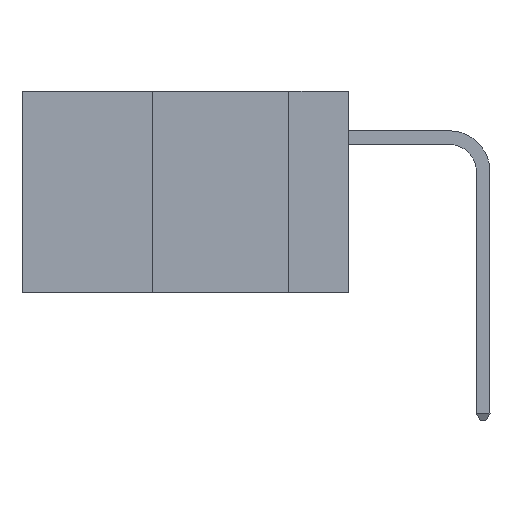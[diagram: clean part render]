
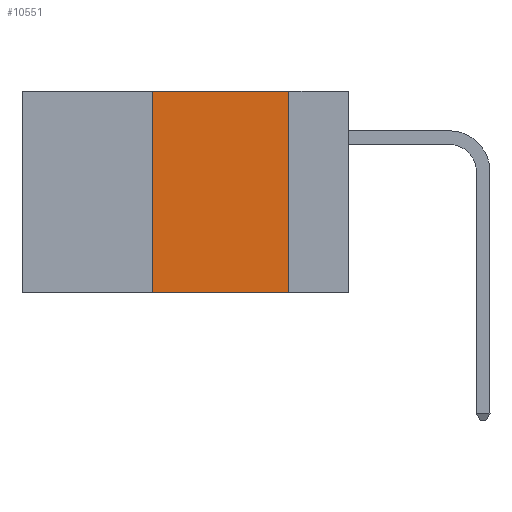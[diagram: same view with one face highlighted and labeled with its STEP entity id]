
A CAD part, left-side view. The second image highlights one B-rep face of the part: STEP entity #10551.
In plain terms, the highlighted planar face has unit normal (-1, 0, 0).
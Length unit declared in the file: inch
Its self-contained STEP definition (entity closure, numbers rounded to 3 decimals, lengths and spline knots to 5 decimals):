
#2004 = VERTEX_POINT ( 'NONE', #26860 ) ;
#2212 = EDGE_CURVE ( 'NONE', #38473, #3203, #31771, .T. ) ;
#3203 = VERTEX_POINT ( 'NONE', #31672 ) ;
#3282 = EDGE_CURVE ( 'NONE', #30031, #2004, #11717, .T. ) ;
#3926 = EDGE_CURVE ( 'NONE', #38473, #30031, #19703, .T. ) ;
#5489 = CARTESIAN_POINT ( 'NONE',  ( 0., 0.11, 0. ) ) ;
#5500 = DIRECTION ( 'NONE',  ( 0., -1., 0. ) ) ;
#5546 = CARTESIAN_POINT ( 'NONE',  ( 0., 0.36, -0.37 ) ) ;
#6443 = PLANE ( 'NONE',  #30149 ) ;
#7255 = ORIENTED_EDGE ( 'NONE', *, *, #3282, .F. ) ;
#7257 = CARTESIAN_POINT ( 'NONE',  ( 0., 0.36, 0. ) ) ;
#8754 = VECTOR ( 'NONE', #25417, 39.37008 ) ;
#10551 = ADVANCED_FACE ( 'NONE', ( #21468 ), #6443, .F. ) ;
#11430 = CARTESIAN_POINT ( 'NONE',  ( 0., 0.6, -0.37 ) ) ;
#11717 = LINE ( 'NONE', #24358, #22481 ) ;
#12381 = CARTESIAN_POINT ( 'NONE',  ( 0., 0.6, 0. ) ) ;
#15226 = ORIENTED_EDGE ( 'NONE', *, *, #2212, .T. ) ;
#18297 = EDGE_LOOP ( 'NONE', ( #26892, #7255, #31265, #15226 ) ) ;
#19703 = LINE ( 'NONE', #7257, #8754 ) ;
#21468 = FACE_OUTER_BOUND ( 'NONE', #18297, .T. ) ;
#21863 = DIRECTION ( 'NONE',  ( 0., 0., -1. ) ) ;
#22481 = VECTOR ( 'NONE', #38576, 39.37008 ) ;
#22729 = CARTESIAN_POINT ( 'NONE',  ( 0., 0.36, 0. ) ) ;
#24358 = CARTESIAN_POINT ( 'NONE',  ( 0., 0.6, 0. ) ) ;
#25417 = DIRECTION ( 'NONE',  ( 0., 0., 1. ) ) ;
#26860 = CARTESIAN_POINT ( 'NONE',  ( 0., 0.11, 0. ) ) ;
#26892 = ORIENTED_EDGE ( 'NONE', *, *, #28267, .F. ) ;
#28267 = EDGE_CURVE ( 'NONE', #2004, #3203, #35875, .T. ) ;
#30031 = VERTEX_POINT ( 'NONE', #22729 ) ;
#30147 = DIRECTION ( 'NONE',  ( 1., 0., 0. ) ) ;
#30149 = AXIS2_PLACEMENT_3D ( 'NONE', #12381, #30147, #21863 ) ;
#31265 = ORIENTED_EDGE ( 'NONE', *, *, #3926, .F. ) ;
#31408 = VECTOR ( 'NONE', #36070, 39.37008 ) ;
#31672 = CARTESIAN_POINT ( 'NONE',  ( 0., 0.11, -0.37 ) ) ;
#31771 = LINE ( 'NONE', #11430, #33510 ) ;
#33510 = VECTOR ( 'NONE', #5500, 39.37008 ) ;
#35875 = LINE ( 'NONE', #5489, #31408 ) ;
#36070 = DIRECTION ( 'NONE',  ( 0., 0., -1. ) ) ;
#38473 = VERTEX_POINT ( 'NONE', #5546 ) ;
#38576 = DIRECTION ( 'NONE',  ( 0., -1., 0. ) ) ;
